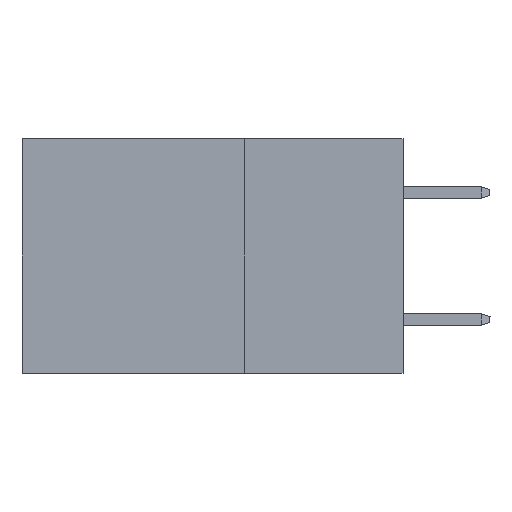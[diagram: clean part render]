
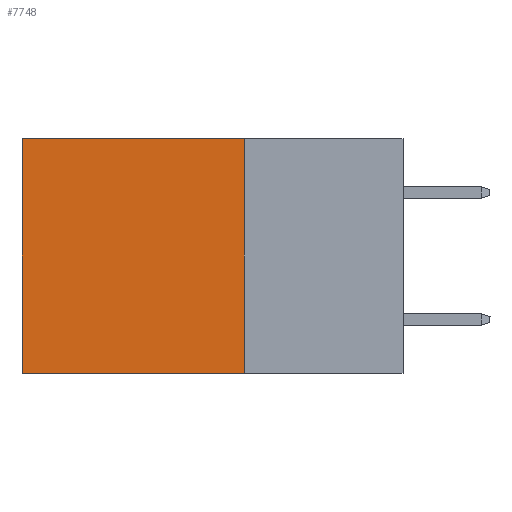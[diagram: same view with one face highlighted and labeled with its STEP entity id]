
A CAD part, left-side view. The second image highlights one B-rep face of the part: STEP entity #7748.
In plain terms, the highlighted planar face has unit normal (-1, 0, 0).
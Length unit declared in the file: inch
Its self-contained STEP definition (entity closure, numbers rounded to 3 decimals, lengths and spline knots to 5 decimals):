
#485 = ORIENTED_EDGE ( 'NONE', *, *, #8123, .T. ) ;
#1719 = CARTESIAN_POINT ( 'NONE',  ( 0.2875, 0.6, 0. ) ) ;
#3671 = LINE ( 'NONE', #8007, #4369 ) ;
#4135 = DIRECTION ( 'NONE',  ( 1., 0., 0. ) ) ;
#4369 = VECTOR ( 'NONE', #24945, 39.37008 ) ;
#4703 = DIRECTION ( 'NONE',  ( 0., 1., 0. ) ) ;
#4850 = ORIENTED_EDGE ( 'NONE', *, *, #27576, .F. ) ;
#4991 = LINE ( 'NONE', #13458, #22317 ) ;
#5663 = CARTESIAN_POINT ( 'NONE',  ( 0.2875, 0.6, -0.37 ) ) ;
#5764 = VERTEX_POINT ( 'NONE', #25066 ) ;
#6611 = EDGE_CURVE ( 'NONE', #5764, #25557, #17416, .T. ) ;
#6683 = CARTESIAN_POINT ( 'NONE',  ( 0.2875, 0.25, -0.37 ) ) ;
#6904 = VECTOR ( 'NONE', #19509, 39.37008 ) ;
#7646 = FACE_OUTER_BOUND ( 'NONE', #7893, .T. ) ;
#7748 = ADVANCED_FACE ( 'NONE', ( #7646 ), #14993, .F. ) ;
#7893 = EDGE_LOOP ( 'NONE', ( #485, #23010, #4850, #12985 ) ) ;
#8007 = CARTESIAN_POINT ( 'NONE',  ( 0.2875, 0.25, 0. ) ) ;
#8123 = EDGE_CURVE ( 'NONE', #14644, #25557, #12401, .T. ) ;
#9700 = AXIS2_PLACEMENT_3D ( 'NONE', #27233, #4135, #27373 ) ;
#11968 = VECTOR ( 'NONE', #18876, 39.37008 ) ;
#12401 = LINE ( 'NONE', #1719, #11968 ) ;
#12581 = VERTEX_POINT ( 'NONE', #13407 ) ;
#12985 = ORIENTED_EDGE ( 'NONE', *, *, #25381, .T. ) ;
#13407 = CARTESIAN_POINT ( 'NONE',  ( 0.2875, 0.25, 0. ) ) ;
#13450 = CARTESIAN_POINT ( 'NONE',  ( 0.2875, 0.6, 0. ) ) ;
#13458 = CARTESIAN_POINT ( 'NONE',  ( 0.2875, 0.25, 0. ) ) ;
#14644 = VERTEX_POINT ( 'NONE', #13450 ) ;
#14993 = PLANE ( 'NONE',  #9700 ) ;
#17416 = LINE ( 'NONE', #6683, #6904 ) ;
#18876 = DIRECTION ( 'NONE',  ( 0., 0., -1. ) ) ;
#19509 = DIRECTION ( 'NONE',  ( 0., 1., 0. ) ) ;
#22317 = VECTOR ( 'NONE', #4703, 39.37008 ) ;
#23010 = ORIENTED_EDGE ( 'NONE', *, *, #6611, .F. ) ;
#24945 = DIRECTION ( 'NONE',  ( 0., 0., -1. ) ) ;
#25066 = CARTESIAN_POINT ( 'NONE',  ( 0.2875, 0.25, -0.37 ) ) ;
#25381 = EDGE_CURVE ( 'NONE', #12581, #14644, #4991, .T. ) ;
#25557 = VERTEX_POINT ( 'NONE', #5663 ) ;
#27233 = CARTESIAN_POINT ( 'NONE',  ( 0.2875, 0.25, 0. ) ) ;
#27373 = DIRECTION ( 'NONE',  ( 0., 0., -1. ) ) ;
#27576 = EDGE_CURVE ( 'NONE', #12581, #5764, #3671, .T. ) ;
